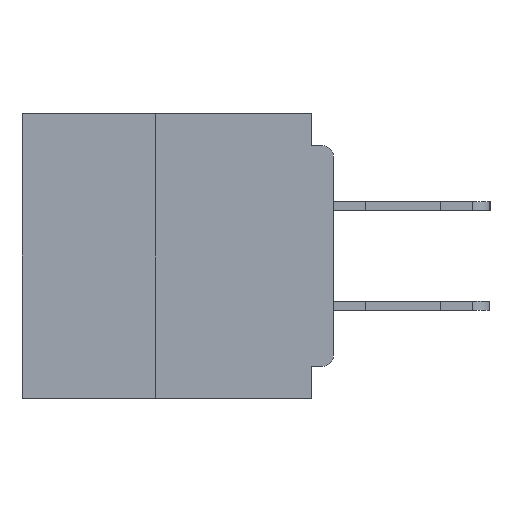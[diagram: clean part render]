
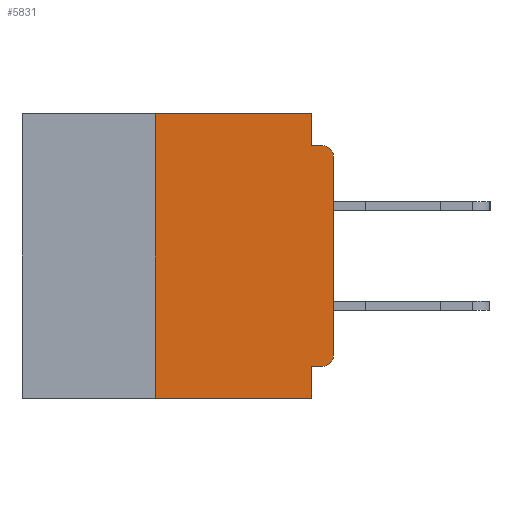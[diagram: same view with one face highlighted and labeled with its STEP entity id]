
A CAD part, left-side view. The second image highlights one B-rep face of the part: STEP entity #5831.
In plain terms, the highlighted planar face has unit normal (-1, 0, 0).
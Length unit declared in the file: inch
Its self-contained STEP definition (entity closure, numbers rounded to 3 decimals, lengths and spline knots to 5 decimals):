
#37 = EDGE_CURVE ( 'NONE', #24859, #57982, #21751, .T. ) ;
#101 = DIRECTION ( 'NONE',  ( 1., 0., 0. ) ) ;
#931 = CARTESIAN_POINT ( 'NONE',  ( 0., 0.015, -0.355 ) ) ;
#1499 = EDGE_CURVE ( 'NONE', #20910, #53045, #3321, .T. ) ;
#1650 = DIRECTION ( 'NONE',  ( 0., -1., 0. ) ) ;
#2727 = DIRECTION ( 'NONE',  ( 0., 0., -1. ) ) ;
#2991 = ORIENTED_EDGE ( 'NONE', *, *, #42220, .F. ) ;
#3321 = LINE ( 'NONE', #49413, #23075 ) ;
#4713 = ORIENTED_EDGE ( 'NONE', *, *, #37, .F. ) ;
#5576 = LINE ( 'NONE', #34871, #28107 ) ;
#5831 = ADVANCED_FACE ( 'NONE', ( #16994 ), #15275, .F. ) ;
#6100 = CARTESIAN_POINT ( 'NONE',  ( 0., 0., -0.06 ) ) ;
#6104 = CARTESIAN_POINT ( 'NONE',  ( 0., 0., 0. ) ) ;
#7467 = ORIENTED_EDGE ( 'NONE', *, *, #22359, .F. ) ;
#9460 = CARTESIAN_POINT ( 'NONE',  ( 0., 0.25, -0.4 ) ) ;
#9823 = AXIS2_PLACEMENT_3D ( 'NONE', #24345, #101, #45700 ) ;
#9904 = VERTEX_POINT ( 'NONE', #55756 ) ;
#10549 = CARTESIAN_POINT ( 'NONE',  ( 0., 0.015, -0.06 ) ) ;
#10580 = ORIENTED_EDGE ( 'NONE', *, *, #11447, .T. ) ;
#10582 = CARTESIAN_POINT ( 'NONE',  ( 0., 0., -0.045 ) ) ;
#10790 = CARTESIAN_POINT ( 'NONE',  ( 0., 0.031, -0.4 ) ) ;
#11337 = VERTEX_POINT ( 'NONE', #52110 ) ;
#11447 = EDGE_CURVE ( 'NONE', #16970, #30874, #23460, .T. ) ;
#12432 = CARTESIAN_POINT ( 'NONE',  ( 0., 0.015, -0.34 ) ) ;
#12457 = ORIENTED_EDGE ( 'NONE', *, *, #56486, .F. ) ;
#13942 = DIRECTION ( 'NONE',  ( 0., 0., 1. ) ) ;
#15039 = DIRECTION ( 'NONE',  ( 0., 0., -1. ) ) ;
#15275 = PLANE ( 'NONE',  #9823 ) ;
#15877 = ORIENTED_EDGE ( 'NONE', *, *, #26120, .T. ) ;
#16939 = DIRECTION ( 'NONE',  ( 0., 0., -1. ) ) ;
#16970 = VERTEX_POINT ( 'NONE', #931 ) ;
#16994 = FACE_OUTER_BOUND ( 'NONE', #24187, .T. ) ;
#18632 = EDGE_CURVE ( 'NONE', #11337, #35617, #5576, .T. ) ;
#19634 = LINE ( 'NONE', #9460, #42238 ) ;
#20497 = CARTESIAN_POINT ( 'NONE',  ( 0., 0., -0.34 ) ) ;
#20910 = VERTEX_POINT ( 'NONE', #39298 ) ;
#21751 = LINE ( 'NONE', #10582, #32297 ) ;
#21807 = AXIS2_PLACEMENT_3D ( 'NONE', #10549, #42071, #15039 ) ;
#22359 = EDGE_CURVE ( 'NONE', #16970, #9904, #24256, .T. ) ;
#22847 = VECTOR ( 'NONE', #31617, 39.37008 ) ;
#23075 = VECTOR ( 'NONE', #48904, 39.37008 ) ;
#23460 = CIRCLE ( 'NONE', #49697, 0.015 ) ;
#23799 = VERTEX_POINT ( 'NONE', #6100 ) ;
#24187 = EDGE_LOOP ( 'NONE', ( #15877, #28595, #4713, #12457, #44810, #36510, #35649, #2991, #7467, #10580 ) ) ;
#24256 = LINE ( 'NONE', #27084, #22847 ) ;
#24345 = CARTESIAN_POINT ( 'NONE',  ( 0., 0.437, 0. ) ) ;
#24621 = CIRCLE ( 'NONE', #21807, 0.015 ) ;
#24859 = VERTEX_POINT ( 'NONE', #49757 ) ;
#26120 = EDGE_CURVE ( 'NONE', #30874, #23799, #53669, .T. ) ;
#26290 = CARTESIAN_POINT ( 'NONE',  ( 0., 0.031, 0. ) ) ;
#27084 = CARTESIAN_POINT ( 'NONE',  ( 0., 0., -0.355 ) ) ;
#28035 = VECTOR ( 'NONE', #2727, 39.37008 ) ;
#28107 = VECTOR ( 'NONE', #53075, 39.37008 ) ;
#28164 = VECTOR ( 'NONE', #53556, 39.37008 ) ;
#28595 = ORIENTED_EDGE ( 'NONE', *, *, #56774, .T. ) ;
#29671 = VECTOR ( 'NONE', #51090, 39.37008 ) ;
#30874 = VERTEX_POINT ( 'NONE', #20497 ) ;
#31617 = DIRECTION ( 'NONE',  ( 0., 1., 0. ) ) ;
#32297 = VECTOR ( 'NONE', #1650, 39.37008 ) ;
#33631 = CARTESIAN_POINT ( 'NONE',  ( 0., 0.015, -0.045 ) ) ;
#34871 = CARTESIAN_POINT ( 'NONE',  ( 0., 0.437, -0.4 ) ) ;
#35617 = VERTEX_POINT ( 'NONE', #10790 ) ;
#35649 = ORIENTED_EDGE ( 'NONE', *, *, #18632, .T. ) ;
#36510 = ORIENTED_EDGE ( 'NONE', *, *, #57753, .F. ) ;
#39298 = CARTESIAN_POINT ( 'NONE',  ( 0., 0.25, 0. ) ) ;
#42071 = DIRECTION ( 'NONE',  ( -1., 0., 0. ) ) ;
#42220 = EDGE_CURVE ( 'NONE', #9904, #35617, #52108, .T. ) ;
#42238 = VECTOR ( 'NONE', #13942, 39.37008 ) ;
#43070 = LINE ( 'NONE', #26290, #28164 ) ;
#44005 = DIRECTION ( 'NONE',  ( -1., 0., 0. ) ) ;
#44810 = ORIENTED_EDGE ( 'NONE', *, *, #1499, .F. ) ;
#45700 = DIRECTION ( 'NONE',  ( 0., 0., -1. ) ) ;
#48904 = DIRECTION ( 'NONE',  ( 0., -1., 0. ) ) ;
#49413 = CARTESIAN_POINT ( 'NONE',  ( 0., 0.437, 0. ) ) ;
#49697 = AXIS2_PLACEMENT_3D ( 'NONE', #12432, #44005, #16939 ) ;
#49757 = CARTESIAN_POINT ( 'NONE',  ( 0., 0.031, -0.045 ) ) ;
#51090 = DIRECTION ( 'NONE',  ( 0., 0., 1. ) ) ;
#51546 = CARTESIAN_POINT ( 'NONE',  ( 0., 0.031, 0. ) ) ;
#52108 = LINE ( 'NONE', #56964, #28035 ) ;
#52110 = CARTESIAN_POINT ( 'NONE',  ( 0., 0.25, -0.4 ) ) ;
#53045 = VERTEX_POINT ( 'NONE', #51546 ) ;
#53075 = DIRECTION ( 'NONE',  ( 0., -1., 0. ) ) ;
#53556 = DIRECTION ( 'NONE',  ( 0., 0., -1. ) ) ;
#53669 = LINE ( 'NONE', #6104, #29671 ) ;
#55756 = CARTESIAN_POINT ( 'NONE',  ( 0., 0.031, -0.355 ) ) ;
#56486 = EDGE_CURVE ( 'NONE', #53045, #24859, #43070, .T. ) ;
#56774 = EDGE_CURVE ( 'NONE', #23799, #57982, #24621, .T. ) ;
#56964 = CARTESIAN_POINT ( 'NONE',  ( 0., 0.031, -0.4 ) ) ;
#57753 = EDGE_CURVE ( 'NONE', #11337, #20910, #19634, .T. ) ;
#57982 = VERTEX_POINT ( 'NONE', #33631 ) ;
